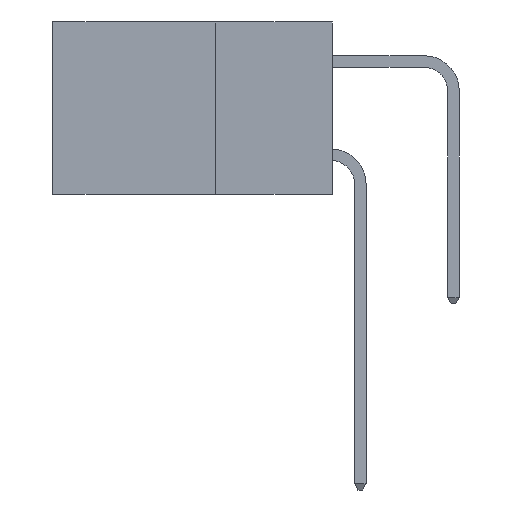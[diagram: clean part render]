
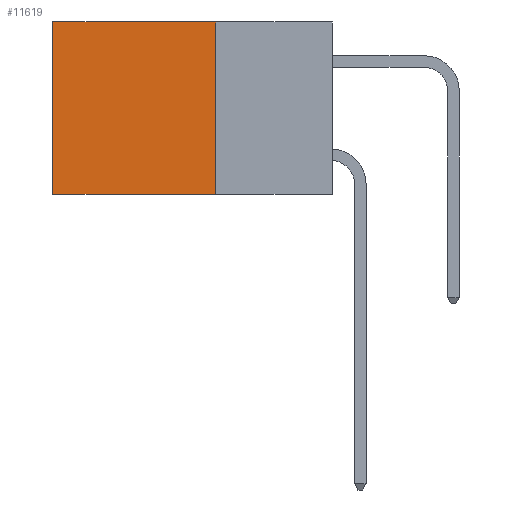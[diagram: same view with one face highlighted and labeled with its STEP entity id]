
A CAD part, left-side view. The second image highlights one B-rep face of the part: STEP entity #11619.
In plain terms, the highlighted planar face has unit normal (-1, 0, 0).
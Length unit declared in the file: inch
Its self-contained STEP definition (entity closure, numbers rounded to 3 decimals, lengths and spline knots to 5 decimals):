
#316 = LINE ( 'NONE', #6926, #7037 ) ;
#569 = DIRECTION ( 'NONE',  ( 0., 0., -1. ) ) ;
#894 = CARTESIAN_POINT ( 'NONE',  ( 0.2615, 0.25, -0.37 ) ) ;
#1215 = DIRECTION ( 'NONE',  ( 0., 0., -1. ) ) ;
#1828 = EDGE_CURVE ( 'NONE', #4535, #14518, #10591, .T. ) ;
#2172 = EDGE_CURVE ( 'NONE', #14518, #8673, #12493, .T. ) ;
#2281 = CARTESIAN_POINT ( 'NONE',  ( 0.2615, 0.25, 0. ) ) ;
#2562 = VECTOR ( 'NONE', #15903, 39.37008 ) ;
#3509 = CARTESIAN_POINT ( 'NONE',  ( 0.2615, 0.6, -0.37 ) ) ;
#3934 = ORIENTED_EDGE ( 'NONE', *, *, #1828, .F. ) ;
#4144 = VECTOR ( 'NONE', #12215, 39.37008 ) ;
#4535 = VERTEX_POINT ( 'NONE', #2281 ) ;
#6185 = VERTEX_POINT ( 'NONE', #9120 ) ;
#6916 = VECTOR ( 'NONE', #569, 39.37008 ) ;
#6926 = CARTESIAN_POINT ( 'NONE',  ( 0.2615, 0.25, 0. ) ) ;
#7037 = VECTOR ( 'NONE', #15558, 39.37008 ) ;
#7484 = PLANE ( 'NONE',  #10126 ) ;
#8673 = VERTEX_POINT ( 'NONE', #10304 ) ;
#8736 = DIRECTION ( 'NONE',  ( 1., 0., 0. ) ) ;
#9120 = CARTESIAN_POINT ( 'NONE',  ( 0.2615, 0.6, 0. ) ) ;
#10126 = AXIS2_PLACEMENT_3D ( 'NONE', #14894, #8736, #1215 ) ;
#10304 = CARTESIAN_POINT ( 'NONE',  ( 0.2615, 0.6, -0.37 ) ) ;
#10377 = LINE ( 'NONE', #3509, #4144 ) ;
#10450 = CARTESIAN_POINT ( 'NONE',  ( 0.2615, 0.25, -0.37 ) ) ;
#10591 = LINE ( 'NONE', #894, #6916 ) ;
#10843 = EDGE_LOOP ( 'NONE', ( #12295, #14510, #3934, #12543 ) ) ;
#11619 = ADVANCED_FACE ( 'NONE', ( #16040 ), #7484, .F. ) ;
#12215 = DIRECTION ( 'NONE',  ( 0., 0., -1. ) ) ;
#12295 = ORIENTED_EDGE ( 'NONE', *, *, #14202, .T. ) ;
#12493 = LINE ( 'NONE', #10450, #2562 ) ;
#12543 = ORIENTED_EDGE ( 'NONE', *, *, #15512, .T. ) ;
#14202 = EDGE_CURVE ( 'NONE', #6185, #8673, #10377, .T. ) ;
#14510 = ORIENTED_EDGE ( 'NONE', *, *, #2172, .F. ) ;
#14518 = VERTEX_POINT ( 'NONE', #14835 ) ;
#14835 = CARTESIAN_POINT ( 'NONE',  ( 0.2615, 0.25, -0.37 ) ) ;
#14894 = CARTESIAN_POINT ( 'NONE',  ( 0.2615, 0.25, -0.37 ) ) ;
#15512 = EDGE_CURVE ( 'NONE', #4535, #6185, #316, .T. ) ;
#15558 = DIRECTION ( 'NONE',  ( 0., 1., 0. ) ) ;
#15903 = DIRECTION ( 'NONE',  ( 0., 1., 0. ) ) ;
#16040 = FACE_OUTER_BOUND ( 'NONE', #10843, .T. ) ;
